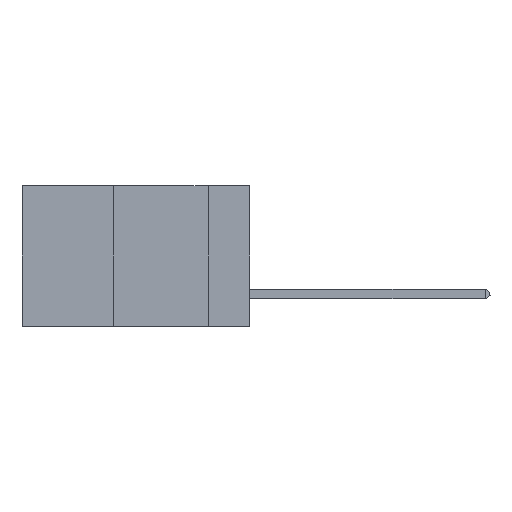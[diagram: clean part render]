
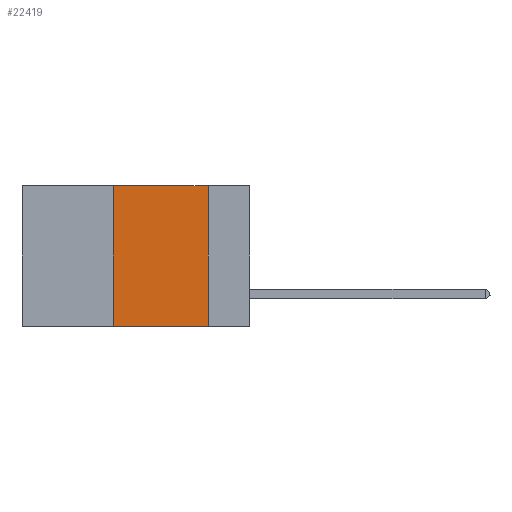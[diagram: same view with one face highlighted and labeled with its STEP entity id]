
A CAD part, left-side view. The second image highlights one B-rep face of the part: STEP entity #22419.
In plain terms, the highlighted planar face has unit normal (-1, 0, 0).
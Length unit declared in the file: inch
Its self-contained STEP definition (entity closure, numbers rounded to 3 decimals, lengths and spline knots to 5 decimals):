
#1605 = DIRECTION ( 'NONE',  ( 0., 0., -1. ) ) ;
#1648 = CARTESIAN_POINT ( 'NONE',  ( 0., 0.11, 0. ) ) ;
#2089 = EDGE_CURVE ( 'NONE', #19391, #23741, #15252, .T. ) ;
#2497 = DIRECTION ( 'NONE',  ( 0., 0., 1. ) ) ;
#3202 = LINE ( 'NONE', #1648, #7923 ) ;
#5423 = ORIENTED_EDGE ( 'NONE', *, *, #7517, .F. ) ;
#5718 = CARTESIAN_POINT ( 'NONE',  ( 0., 0.6, 0. ) ) ;
#5903 = VECTOR ( 'NONE', #15765, 39.37008 ) ;
#6256 = CARTESIAN_POINT ( 'NONE',  ( 0., 0.6, 0. ) ) ;
#6732 = AXIS2_PLACEMENT_3D ( 'NONE', #5718, #16939, #1605 ) ;
#6820 = CARTESIAN_POINT ( 'NONE',  ( 0., 0.11, 0. ) ) ;
#7517 = EDGE_CURVE ( 'NONE', #13313, #23741, #3202, .T. ) ;
#7923 = VECTOR ( 'NONE', #13067, 39.37008 ) ;
#10040 = LINE ( 'NONE', #6256, #5903 ) ;
#10198 = ORIENTED_EDGE ( 'NONE', *, *, #14269, .F. ) ;
#10990 = CARTESIAN_POINT ( 'NONE',  ( 0., 0.6, -0.37 ) ) ;
#13067 = DIRECTION ( 'NONE',  ( 0., 0., -1. ) ) ;
#13165 = DIRECTION ( 'NONE',  ( 0., -1., 0. ) ) ;
#13313 = VERTEX_POINT ( 'NONE', #6820 ) ;
#13662 = CARTESIAN_POINT ( 'NONE',  ( 0., 0.36, 0. ) ) ;
#13790 = VECTOR ( 'NONE', #13165, 39.37008 ) ;
#14015 = VERTEX_POINT ( 'NONE', #22203 ) ;
#14269 = EDGE_CURVE ( 'NONE', #19391, #14015, #22184, .T. ) ;
#15252 = LINE ( 'NONE', #10990, #13790 ) ;
#15424 = ORIENTED_EDGE ( 'NONE', *, *, #19221, .F. ) ;
#15765 = DIRECTION ( 'NONE',  ( 0., -1., 0. ) ) ;
#16939 = DIRECTION ( 'NONE',  ( 1., 0., 0. ) ) ;
#17030 = CARTESIAN_POINT ( 'NONE',  ( 0., 0.36, -0.37 ) ) ;
#17223 = VECTOR ( 'NONE', #2497, 39.37008 ) ;
#17710 = ORIENTED_EDGE ( 'NONE', *, *, #2089, .T. ) ;
#18657 = PLANE ( 'NONE',  #6732 ) ;
#18676 = EDGE_LOOP ( 'NONE', ( #5423, #15424, #10198, #17710 ) ) ;
#18793 = FACE_OUTER_BOUND ( 'NONE', #18676, .T. ) ;
#19221 = EDGE_CURVE ( 'NONE', #14015, #13313, #10040, .T. ) ;
#19391 = VERTEX_POINT ( 'NONE', #17030 ) ;
#22184 = LINE ( 'NONE', #13662, #17223 ) ;
#22203 = CARTESIAN_POINT ( 'NONE',  ( 0., 0.36, 0. ) ) ;
#22419 = ADVANCED_FACE ( 'NONE', ( #18793 ), #18657, .F. ) ;
#23161 = CARTESIAN_POINT ( 'NONE',  ( 0., 0.11, -0.37 ) ) ;
#23741 = VERTEX_POINT ( 'NONE', #23161 ) ;
